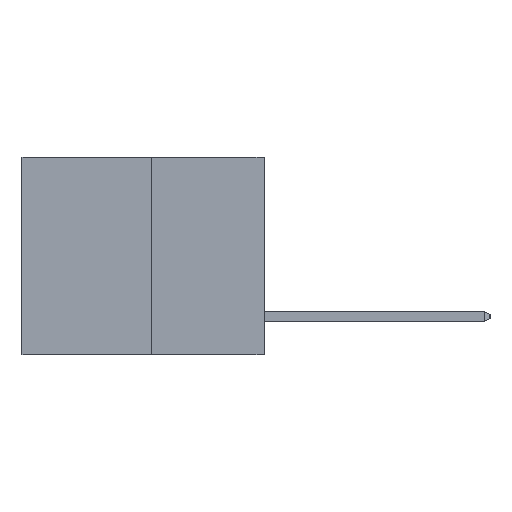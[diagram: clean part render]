
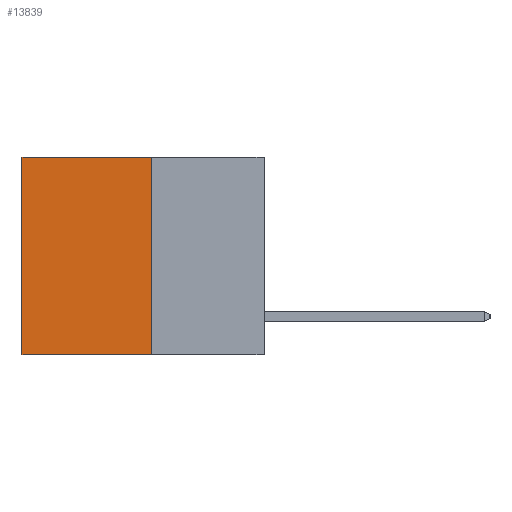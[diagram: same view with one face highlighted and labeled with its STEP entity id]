
A CAD part, left-side view. The second image highlights one B-rep face of the part: STEP entity #13839.
In plain terms, the highlighted planar face has unit normal (-1, 0, 0).
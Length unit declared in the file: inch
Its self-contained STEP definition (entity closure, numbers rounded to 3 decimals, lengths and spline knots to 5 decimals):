
#1034 = LINE ( 'NONE', #12671, #12368 ) ;
#1722 = LINE ( 'NONE', #17780, #11336 ) ;
#2458 = LINE ( 'NONE', #15326, #5922 ) ;
#2590 = PLANE ( 'NONE',  #14322 ) ;
#2703 = VERTEX_POINT ( 'NONE', #9205 ) ;
#3681 = ORIENTED_EDGE ( 'NONE', *, *, #12645, .F. ) ;
#4118 = DIRECTION ( 'NONE',  ( 1., 0., 0. ) ) ;
#4235 = DIRECTION ( 'NONE',  ( 0., 0., -1. ) ) ;
#5895 = CARTESIAN_POINT ( 'NONE',  ( 0.3165, 0.28, 0. ) ) ;
#5922 = VECTOR ( 'NONE', #7400, 39.37008 ) ;
#6579 = CARTESIAN_POINT ( 'NONE',  ( 0.3165, 0.28, 0. ) ) ;
#7400 = DIRECTION ( 'NONE',  ( 0., 0., -1. ) ) ;
#7597 = EDGE_CURVE ( 'NONE', #10015, #20195, #2458, .T. ) ;
#8971 = CARTESIAN_POINT ( 'NONE',  ( 0.3165, 0.28, -0.49 ) ) ;
#9205 = CARTESIAN_POINT ( 'NONE',  ( 0.3165, 0.6, 0. ) ) ;
#9352 = FACE_OUTER_BOUND ( 'NONE', #18362, .T. ) ;
#9430 = VERTEX_POINT ( 'NONE', #11434 ) ;
#10015 = VERTEX_POINT ( 'NONE', #6579 ) ;
#10327 = VECTOR ( 'NONE', #19933, 39.37008 ) ;
#11336 = VECTOR ( 'NONE', #16256, 39.37008 ) ;
#11434 = CARTESIAN_POINT ( 'NONE',  ( 0.3165, 0.6, -0.49 ) ) ;
#11465 = CARTESIAN_POINT ( 'NONE',  ( 0.3165, 0.28, -0.49 ) ) ;
#11556 = LINE ( 'NONE', #5895, #10327 ) ;
#12368 = VECTOR ( 'NONE', #15845, 39.37008 ) ;
#12620 = ORIENTED_EDGE ( 'NONE', *, *, #7597, .F. ) ;
#12645 = EDGE_CURVE ( 'NONE', #20195, #9430, #1034, .T. ) ;
#12671 = CARTESIAN_POINT ( 'NONE',  ( 0.3165, 0.28, -0.49 ) ) ;
#13202 = ORIENTED_EDGE ( 'NONE', *, *, #13901, .T. ) ;
#13839 = ADVANCED_FACE ( 'NONE', ( #9352 ), #2590, .F. ) ;
#13901 = EDGE_CURVE ( 'NONE', #10015, #2703, #11556, .T. ) ;
#14092 = EDGE_CURVE ( 'NONE', #2703, #9430, #1722, .T. ) ;
#14322 = AXIS2_PLACEMENT_3D ( 'NONE', #8971, #4118, #4235 ) ;
#15326 = CARTESIAN_POINT ( 'NONE',  ( 0.3165, 0.28, -0.49 ) ) ;
#15845 = DIRECTION ( 'NONE',  ( 0., 1., 0. ) ) ;
#16256 = DIRECTION ( 'NONE',  ( 0., 0., -1. ) ) ;
#16290 = ORIENTED_EDGE ( 'NONE', *, *, #14092, .T. ) ;
#17780 = CARTESIAN_POINT ( 'NONE',  ( 0.3165, 0.6, -0.49 ) ) ;
#18362 = EDGE_LOOP ( 'NONE', ( #16290, #3681, #12620, #13202 ) ) ;
#19933 = DIRECTION ( 'NONE',  ( 0., 1., 0. ) ) ;
#20195 = VERTEX_POINT ( 'NONE', #11465 ) ;
